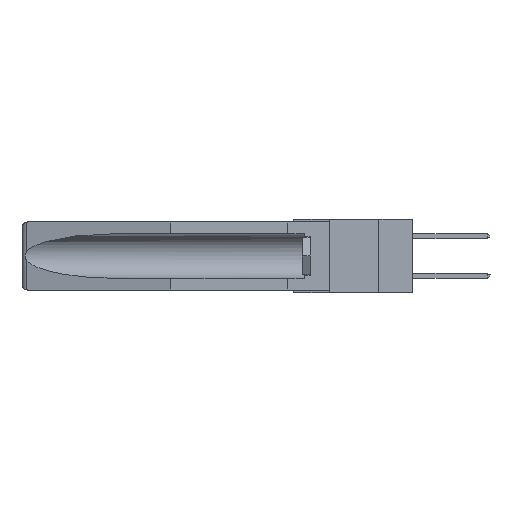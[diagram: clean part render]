
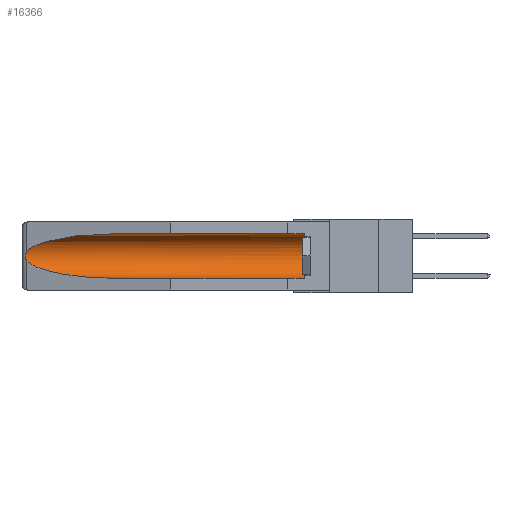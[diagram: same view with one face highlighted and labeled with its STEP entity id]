
A CAD part, left-side view. The second image highlights one B-rep face of the part: STEP entity #16366.
In plain terms, the highlighted cylindrical face has radius 2.857 mm (diameter 5.715 mm), a partial arc.
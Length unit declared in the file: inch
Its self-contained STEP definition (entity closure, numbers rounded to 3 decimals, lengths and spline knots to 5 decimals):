
#59 = DIRECTION ( 'NONE',  ( 0., 1., 0. ) ) ;
#165 = CARTESIAN_POINT ( 'NONE',  ( 0.155, 1.07973, -0.059 ) ) ;
#315 = LINE ( 'NONE', #2381, #12454 ) ;
#487 = CARTESIAN_POINT ( 'NONE',  ( 0.155, 1.07973, -0.284 ) ) ;
#781 = CARTESIAN_POINT ( 'NONE',  ( 0.155, 1.07973, -0.059 ) ) ;
#2381 = CARTESIAN_POINT ( 'NONE',  ( 0.155, -0.30754, -0.059 ) ) ;
#2599 = VERTEX_POINT ( 'NONE', #165 ) ;
#4305 = EDGE_CURVE ( 'NONE', #2599, #26112, #12811, .T. ) ;
#4951 = DIRECTION ( 'NONE',  ( 0., 1., 0. ) ) ;
#5461 = DIRECTION ( 'NONE',  ( 0., -1., 0. ) ) ;
#5746 = EDGE_LOOP ( 'NONE', ( #6849, #10615, #7622, #22642, #24907, #9301 ) ) ;
#6849 = ORIENTED_EDGE ( 'NONE', *, *, #4305, .T. ) ;
#7283 = DIRECTION ( 'NONE',  ( 0., 1., 0. ) ) ;
#7376 = CARTESIAN_POINT ( 'NONE',  ( 0.26537, 1.52718, -0.14972 ) ) ;
#7622 = ORIENTED_EDGE ( 'NONE', *, *, #22863, .T. ) ;
#7949 = EDGE_CURVE ( 'NONE', #26654, #2599, #315, .T. ) ;
#8041 = CARTESIAN_POINT ( 'NONE',  ( 0.26537, 1.52718, -0.14972 ) ) ;
#9301 = ORIENTED_EDGE ( 'NONE', *, *, #7949, .T. ) ;
#9754 = VECTOR ( 'NONE', #4951, 39.37008 ) ;
#9902 = B_SPLINE_CURVE_WITH_KNOTS ( 'NONE', 3,
 ( #8041, #27469, #11352, #28305, #11138, #11033, #20573, #16191, #20678, #30449 ),
 .UNSPECIFIED., .F., .F.,
 ( 4, 2, 2, 2, 4 ),
 ( 0., 0.00029, 0.00058, 0.00087, 0.00117 ),
 .UNSPECIFIED. ) ;
#10135 = CARTESIAN_POINT ( 'NONE',  ( 0.21114, 1.30732, -0.284 ) ) ;
#10521 = LINE ( 'NONE', #18936, #9754 ) ;
#10615 = ORIENTED_EDGE ( 'NONE', *, *, #10630, .T. ) ;
#10630 = EDGE_CURVE ( 'NONE', #26112, #11671, #9902, .T. ) ;
#11033 = CARTESIAN_POINT ( 'NONE',  ( 0.2675, 1.53308, -0.17534 ) ) ;
#11138 = CARTESIAN_POINT ( 'NONE',  ( 0.2675, 1.53308, -0.16763 ) ) ;
#11310 = CARTESIAN_POINT ( 'NONE',  ( 0.155, 0.126, -0.284 ) ) ;
#11352 = CARTESIAN_POINT ( 'NONE',  ( 0.26654, 1.53092, -0.15636 ) ) ;
#11671 = VERTEX_POINT ( 'NONE', #11687 ) ;
#11687 = CARTESIAN_POINT ( 'NONE',  ( 0.26537, 1.52718, -0.19328 ) ) ;
#12454 = VECTOR ( 'NONE', #59, 39.37008 ) ;
#12734 = DIRECTION ( 'NONE',  ( 0., 0., 1. ) ) ;
#12811 =( BOUNDED_CURVE ( )  B_SPLINE_CURVE ( 3, ( #781, #17696, #22716, #24941 ),
 .UNSPECIFIED., .F., .F. ) 
 B_SPLINE_CURVE_WITH_KNOTS ( ( 4, 4 ),
 ( 4.71239, 6.08839 ),
 .UNSPECIFIED. ) 
 CURVE ( )  GEOMETRIC_REPRESENTATION_ITEM ( )  RATIONAL_B_SPLINE_CURVE ( ( 1., 0.848, 0.848, 1. ) ) 
 REPRESENTATION_ITEM ( '' )  );
#13153 = VERTEX_POINT ( 'NONE', #11310 ) ;
#13460 = CARTESIAN_POINT ( 'NONE',  ( 0.155, 0.126, -0.059 ) ) ;
#13905 = EDGE_CURVE ( 'NONE', #13153, #27376, #10521, .T. ) ;
#15715 = EDGE_CURVE ( 'NONE', #13153, #26654, #18697, .T. ) ;
#16101 =( BOUNDED_CURVE ( )  B_SPLINE_CURVE ( 3, ( #22104, #17397, #10135, #487 ),
 .UNSPECIFIED., .F., .F. ) 
 B_SPLINE_CURVE_WITH_KNOTS ( ( 4, 4 ),
 ( 0.1948, 1.5708 ),
 .UNSPECIFIED. ) 
 CURVE ( )  GEOMETRIC_REPRESENTATION_ITEM ( )  RATIONAL_B_SPLINE_CURVE ( ( 1., 0.848, 0.848, 1. ) ) 
 REPRESENTATION_ITEM ( '' )  );
#16191 = CARTESIAN_POINT ( 'NONE',  ( 0.26655, 1.53094, -0.18657 ) ) ;
#16366 = ADVANCED_FACE ( 'NONE', ( #22027 ), #25081, .F. ) ;
#16741 = DIRECTION ( 'NONE',  ( 0., 0., 1. ) ) ;
#17397 = CARTESIAN_POINT ( 'NONE',  ( 0.25451, 1.48313, -0.24835 ) ) ;
#17571 = CARTESIAN_POINT ( 'NONE',  ( 0.155, 0.126, -0.1715 ) ) ;
#17696 = CARTESIAN_POINT ( 'NONE',  ( 0.21114, 1.30732, -0.059 ) ) ;
#18033 = AXIS2_PLACEMENT_3D ( 'NONE', #17571, #5461, #12734 ) ;
#18697 = CIRCLE ( 'NONE', #18033, 0.1125 ) ;
#18936 = CARTESIAN_POINT ( 'NONE',  ( 0.155, -0.30754, -0.284 ) ) ;
#20573 = CARTESIAN_POINT ( 'NONE',  ( 0.2673, 1.53269, -0.17917 ) ) ;
#20678 = CARTESIAN_POINT ( 'NONE',  ( 0.26597, 1.5296, -0.19026 ) ) ;
#22027 = FACE_OUTER_BOUND ( 'NONE', #5746, .T. ) ;
#22104 = CARTESIAN_POINT ( 'NONE',  ( 0.26537, 1.52718, -0.19328 ) ) ;
#22642 = ORIENTED_EDGE ( 'NONE', *, *, #13905, .F. ) ;
#22716 = CARTESIAN_POINT ( 'NONE',  ( 0.25451, 1.48313, -0.09465 ) ) ;
#22863 = EDGE_CURVE ( 'NONE', #11671, #27376, #16101, .T. ) ;
#23452 = AXIS2_PLACEMENT_3D ( 'NONE', #26734, #7283, #16741 ) ;
#23952 = CARTESIAN_POINT ( 'NONE',  ( 0.155, 1.07973, -0.284 ) ) ;
#24907 = ORIENTED_EDGE ( 'NONE', *, *, #15715, .T. ) ;
#24941 = CARTESIAN_POINT ( 'NONE',  ( 0.26537, 1.52718, -0.14972 ) ) ;
#25081 = CYLINDRICAL_SURFACE ( 'NONE', #23452, 0.1125 ) ;
#26112 = VERTEX_POINT ( 'NONE', #7376 ) ;
#26654 = VERTEX_POINT ( 'NONE', #13460 ) ;
#26734 = CARTESIAN_POINT ( 'NONE',  ( 0.155, -0.30754, -0.1715 ) ) ;
#27376 = VERTEX_POINT ( 'NONE', #23952 ) ;
#27469 = CARTESIAN_POINT ( 'NONE',  ( 0.26597, 1.52961, -0.15275 ) ) ;
#28305 = CARTESIAN_POINT ( 'NONE',  ( 0.2673, 1.5327, -0.16383 ) ) ;
#30449 = CARTESIAN_POINT ( 'NONE',  ( 0.26537, 1.52718, -0.19328 ) ) ;
